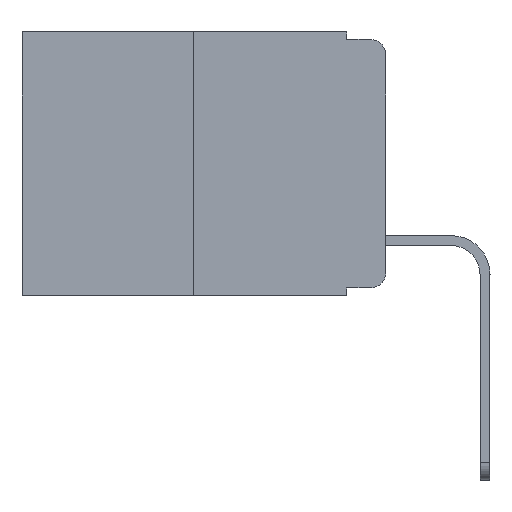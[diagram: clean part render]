
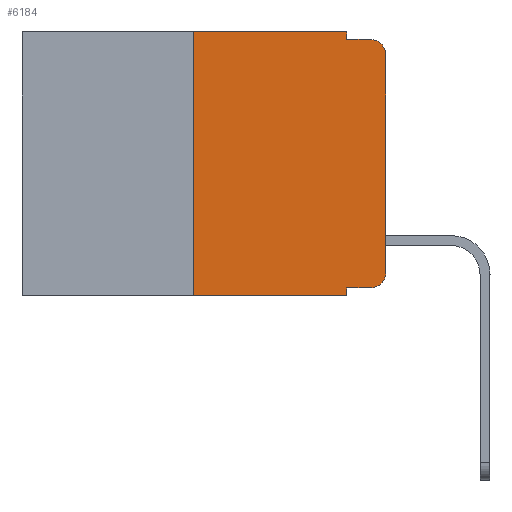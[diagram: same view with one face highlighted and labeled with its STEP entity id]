
A CAD part, left-side view. The second image highlights one B-rep face of the part: STEP entity #6184.
In plain terms, the highlighted planar face has unit normal (-1, 0, 0).
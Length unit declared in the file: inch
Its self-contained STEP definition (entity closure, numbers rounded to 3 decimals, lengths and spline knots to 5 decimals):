
#24 = CARTESIAN_POINT ( 'NONE',  ( 0., 0.051, -0.343 ) ) ;
#350 = ORIENTED_EDGE ( 'NONE', *, *, #4355, .F. ) ;
#774 = VECTOR ( 'NONE', #12443, 39.37008 ) ;
#868 = CARTESIAN_POINT ( 'NONE',  ( 0., 0.25, 0. ) ) ;
#1144 = LINE ( 'NONE', #1861, #774 ) ;
#1433 = DIRECTION ( 'NONE',  ( 0., 0., 1. ) ) ;
#1466 = VERTEX_POINT ( 'NONE', #24 ) ;
#1808 = CARTESIAN_POINT ( 'NONE',  ( 0., 0.473, -0.343 ) ) ;
#1861 = CARTESIAN_POINT ( 'NONE',  ( 0., 0.051, -0.01 ) ) ;
#2335 = VERTEX_POINT ( 'NONE', #13264 ) ;
#2460 = CARTESIAN_POINT ( 'NONE',  ( 0., 0., -0.03 ) ) ;
#2476 = DIRECTION ( 'NONE',  ( 0., 0., -1. ) ) ;
#2513 = LINE ( 'NONE', #13697, #14683 ) ;
#2531 = EDGE_CURVE ( 'NONE', #5516, #6613, #14473, .T. ) ;
#3074 = VERTEX_POINT ( 'NONE', #13747 ) ;
#3075 = LINE ( 'NONE', #14223, #8260 ) ;
#3282 = FACE_OUTER_BOUND ( 'NONE', #8689, .T. ) ;
#4266 = LINE ( 'NONE', #10606, #10555 ) ;
#4355 = EDGE_CURVE ( 'NONE', #3074, #6613, #1144, .T. ) ;
#4395 = AXIS2_PLACEMENT_3D ( 'NONE', #12795, #10344, #7900 ) ;
#4712 = CARTESIAN_POINT ( 'NONE',  ( 0., 0., 0. ) ) ;
#4812 = CARTESIAN_POINT ( 'NONE',  ( 0., 0.25, 0. ) ) ;
#4945 = CARTESIAN_POINT ( 'NONE',  ( 0., 0.051, -0.333 ) ) ;
#5112 = ORIENTED_EDGE ( 'NONE', *, *, #10634, .F. ) ;
#5334 = ORIENTED_EDGE ( 'NONE', *, *, #8831, .T. ) ;
#5512 = VERTEX_POINT ( 'NONE', #7200 ) ;
#5515 = VECTOR ( 'NONE', #13284, 39.37008 ) ;
#5516 = VERTEX_POINT ( 'NONE', #2460 ) ;
#5745 = ORIENTED_EDGE ( 'NONE', *, *, #2531, .T. ) ;
#5947 = CARTESIAN_POINT ( 'NONE',  ( 0., 0.473, 0. ) ) ;
#6056 = DIRECTION ( 'NONE',  ( 0., 0., -1. ) ) ;
#6184 = ADVANCED_FACE ( 'NONE', ( #3282 ), #9602, .F. ) ;
#6289 = LINE ( 'NONE', #4812, #8300 ) ;
#6446 = CARTESIAN_POINT ( 'NONE',  ( 0., 0.02, -0.313 ) ) ;
#6460 = AXIS2_PLACEMENT_3D ( 'NONE', #5947, #7185, #6056 ) ;
#6613 = VERTEX_POINT ( 'NONE', #12845 ) ;
#6685 = VERTEX_POINT ( 'NONE', #4945 ) ;
#7013 = EDGE_CURVE ( 'NONE', #5512, #1466, #9356, .T. ) ;
#7185 = DIRECTION ( 'NONE',  ( 1., 0., 0. ) ) ;
#7200 = CARTESIAN_POINT ( 'NONE',  ( 0., 0.25, -0.343 ) ) ;
#7391 = LINE ( 'NONE', #8587, #5515 ) ;
#7622 = EDGE_CURVE ( 'NONE', #6685, #12483, #2513, .T. ) ;
#7730 = VERTEX_POINT ( 'NONE', #868 ) ;
#7900 = DIRECTION ( 'NONE',  ( 0., 0., -1. ) ) ;
#8198 = DIRECTION ( 'NONE',  ( 0., 0., 1. ) ) ;
#8260 = VECTOR ( 'NONE', #2476, 39.37008 ) ;
#8300 = VECTOR ( 'NONE', #1433, 39.37008 ) ;
#8587 = CARTESIAN_POINT ( 'NONE',  ( 0., 0.051, 0. ) ) ;
#8689 = EDGE_LOOP ( 'NONE', ( #5334, #5745, #350, #9913, #5112, #9243, #9827, #14540, #10484, #11752 ) ) ;
#8831 = EDGE_CURVE ( 'NONE', #11379, #5516, #12257, .T. ) ;
#9243 = ORIENTED_EDGE ( 'NONE', *, *, #12406, .F. ) ;
#9356 = LINE ( 'NONE', #1808, #14712 ) ;
#9602 = PLANE ( 'NONE',  #6460 ) ;
#9827 = ORIENTED_EDGE ( 'NONE', *, *, #7013, .T. ) ;
#9885 = DIRECTION ( 'NONE',  ( -1., 0., 0. ) ) ;
#9913 = ORIENTED_EDGE ( 'NONE', *, *, #12498, .F. ) ;
#10344 = DIRECTION ( 'NONE',  ( -1., 0., 0. ) ) ;
#10484 = ORIENTED_EDGE ( 'NONE', *, *, #7622, .T. ) ;
#10555 = VECTOR ( 'NONE', #11851, 39.37008 ) ;
#10606 = CARTESIAN_POINT ( 'NONE',  ( 0., 0.473, 0. ) ) ;
#10634 = EDGE_CURVE ( 'NONE', #7730, #2335, #4266, .T. ) ;
#10965 = AXIS2_PLACEMENT_3D ( 'NONE', #6446, #9885, #14632 ) ;
#11128 = VECTOR ( 'NONE', #8198, 39.37008 ) ;
#11176 = CARTESIAN_POINT ( 'NONE',  ( 0., 0., -0.313 ) ) ;
#11322 = DIRECTION ( 'NONE',  ( 0., -1., 0. ) ) ;
#11379 = VERTEX_POINT ( 'NONE', #11176 ) ;
#11752 = ORIENTED_EDGE ( 'NONE', *, *, #13599, .T. ) ;
#11851 = DIRECTION ( 'NONE',  ( 0., -1., 0. ) ) ;
#12095 = CARTESIAN_POINT ( 'NONE',  ( 0., 0.02, -0.333 ) ) ;
#12257 = LINE ( 'NONE', #4712, #11128 ) ;
#12406 = EDGE_CURVE ( 'NONE', #5512, #7730, #6289, .T. ) ;
#12443 = DIRECTION ( 'NONE',  ( 0., -1., 0. ) ) ;
#12483 = VERTEX_POINT ( 'NONE', #12095 ) ;
#12498 = EDGE_CURVE ( 'NONE', #2335, #3074, #7391, .T. ) ;
#12795 = CARTESIAN_POINT ( 'NONE',  ( 0., 0.02, -0.03 ) ) ;
#12845 = CARTESIAN_POINT ( 'NONE',  ( 0., 0.02, -0.01 ) ) ;
#13264 = CARTESIAN_POINT ( 'NONE',  ( 0., 0.051, 0. ) ) ;
#13284 = DIRECTION ( 'NONE',  ( 0., 0., -1. ) ) ;
#13599 = EDGE_CURVE ( 'NONE', #12483, #11379, #14897, .T. ) ;
#13646 = DIRECTION ( 'NONE',  ( 0., -1., 0. ) ) ;
#13697 = CARTESIAN_POINT ( 'NONE',  ( 0., 0.051, -0.333 ) ) ;
#13747 = CARTESIAN_POINT ( 'NONE',  ( 0., 0.051, -0.01 ) ) ;
#13992 = EDGE_CURVE ( 'NONE', #6685, #1466, #3075, .T. ) ;
#14223 = CARTESIAN_POINT ( 'NONE',  ( 0., 0.051, 0. ) ) ;
#14473 = CIRCLE ( 'NONE', #4395, 0.02 ) ;
#14540 = ORIENTED_EDGE ( 'NONE', *, *, #13992, .F. ) ;
#14632 = DIRECTION ( 'NONE',  ( 0., 0., -1. ) ) ;
#14683 = VECTOR ( 'NONE', #13646, 39.37008 ) ;
#14712 = VECTOR ( 'NONE', #11322, 39.37008 ) ;
#14897 = CIRCLE ( 'NONE', #10965, 0.02 ) ;
